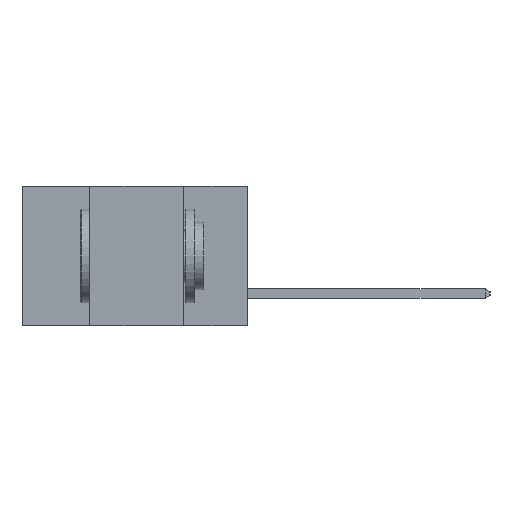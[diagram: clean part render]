
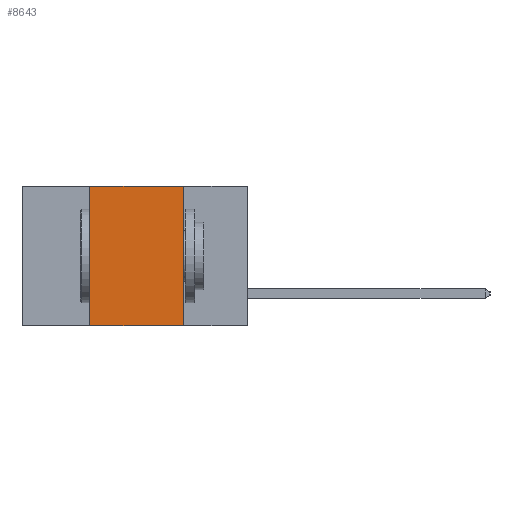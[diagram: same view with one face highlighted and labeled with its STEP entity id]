
A CAD part, left-side view. The second image highlights one B-rep face of the part: STEP entity #8643.
In plain terms, the highlighted planar face has unit normal (-1, 0, 0).
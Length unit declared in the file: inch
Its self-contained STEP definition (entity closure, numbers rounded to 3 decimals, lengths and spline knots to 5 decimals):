
#36 = CARTESIAN_POINT ( 'NONE',  ( 0., 0.17, -0.37 ) ) ;
#85 = EDGE_CURVE ( 'NONE', #2310, #8835, #8907, .T. ) ;
#319 = AXIS2_PLACEMENT_3D ( 'NONE', #9628, #677, #6486 ) ;
#441 = VECTOR ( 'NONE', #4682, 39.37008 ) ;
#677 = DIRECTION ( 'NONE',  ( 1., 0., 0. ) ) ;
#1169 = VECTOR ( 'NONE', #4868, 39.37008 ) ;
#1567 = CARTESIAN_POINT ( 'NONE',  ( 0., 0.42, 0. ) ) ;
#2310 = VERTEX_POINT ( 'NONE', #1567 ) ;
#3093 = ORIENTED_EDGE ( 'NONE', *, *, #85, .F. ) ;
#3168 = ORIENTED_EDGE ( 'NONE', *, *, #9503, .F. ) ;
#3402 = CARTESIAN_POINT ( 'NONE',  ( 0., 0.42, -0.37 ) ) ;
#3533 = CARTESIAN_POINT ( 'NONE',  ( 0., 0.17, -0.37 ) ) ;
#4252 = CARTESIAN_POINT ( 'NONE',  ( 0., 0.17, 0. ) ) ;
#4627 = EDGE_LOOP ( 'NONE', ( #3168, #3093, #8424, #4866 ) ) ;
#4682 = DIRECTION ( 'NONE',  ( 0., 0., 1. ) ) ;
#4866 = ORIENTED_EDGE ( 'NONE', *, *, #9368, .T. ) ;
#4868 = DIRECTION ( 'NONE',  ( 0., -1., 0. ) ) ;
#5166 = CARTESIAN_POINT ( 'NONE',  ( 0., 0.6, 0. ) ) ;
#5962 = VECTOR ( 'NONE', #7526, 39.37008 ) ;
#6486 = DIRECTION ( 'NONE',  ( 0., 0., -1. ) ) ;
#7044 = VERTEX_POINT ( 'NONE', #3533 ) ;
#7094 = LINE ( 'NONE', #9518, #441 ) ;
#7214 = LINE ( 'NONE', #8969, #1169 ) ;
#7526 = DIRECTION ( 'NONE',  ( 0., 0., -1. ) ) ;
#8424 = ORIENTED_EDGE ( 'NONE', *, *, #9173, .F. ) ;
#8616 = FACE_OUTER_BOUND ( 'NONE', #4627, .T. ) ;
#8643 = ADVANCED_FACE ( 'NONE', ( #8616 ), #9661, .F. ) ;
#8666 = VECTOR ( 'NONE', #8674, 39.37008 ) ;
#8674 = DIRECTION ( 'NONE',  ( 0., -1., 0. ) ) ;
#8835 = VERTEX_POINT ( 'NONE', #4252 ) ;
#8907 = LINE ( 'NONE', #5166, #8666 ) ;
#8969 = CARTESIAN_POINT ( 'NONE',  ( 0., 0.6, -0.37 ) ) ;
#9173 = EDGE_CURVE ( 'NONE', #9486, #2310, #7094, .T. ) ;
#9368 = EDGE_CURVE ( 'NONE', #9486, #7044, #7214, .T. ) ;
#9486 = VERTEX_POINT ( 'NONE', #3402 ) ;
#9503 = EDGE_CURVE ( 'NONE', #8835, #7044, #9928, .T. ) ;
#9518 = CARTESIAN_POINT ( 'NONE',  ( 0., 0.42, -0.37 ) ) ;
#9628 = CARTESIAN_POINT ( 'NONE',  ( 0., 0.6, 0. ) ) ;
#9661 = PLANE ( 'NONE',  #319 ) ;
#9928 = LINE ( 'NONE', #36, #5962 ) ;
